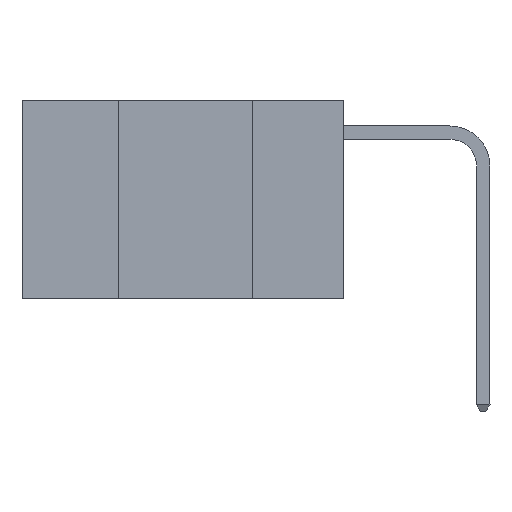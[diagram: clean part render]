
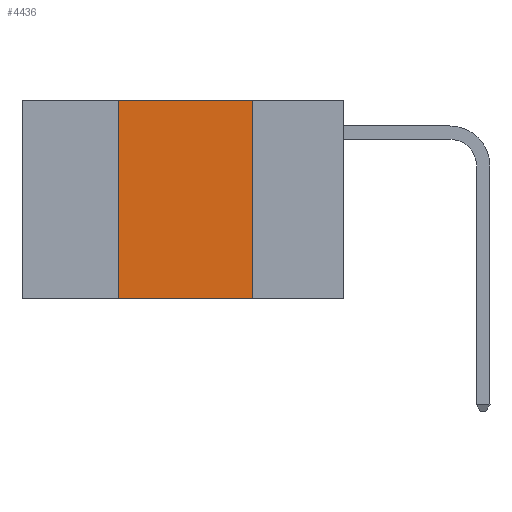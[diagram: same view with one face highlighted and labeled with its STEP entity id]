
A CAD part, left-side view. The second image highlights one B-rep face of the part: STEP entity #4436.
In plain terms, the highlighted planar face has unit normal (-1, 0, 0).
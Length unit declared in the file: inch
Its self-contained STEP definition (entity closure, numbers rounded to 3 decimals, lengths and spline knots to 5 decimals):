
#454 = VECTOR ( 'NONE', #3137, 39.37008 ) ;
#1437 = ORIENTED_EDGE ( 'NONE', *, *, #11161, .F. ) ;
#1546 = DIRECTION ( 'NONE',  ( 1., 0., 0. ) ) ;
#2409 = CARTESIAN_POINT ( 'NONE',  ( 0., 0.6, 0. ) ) ;
#3137 = DIRECTION ( 'NONE',  ( 0., 0., -1. ) ) ;
#3582 = PLANE ( 'NONE',  #13447 ) ;
#3791 = EDGE_CURVE ( 'NONE', #14236, #11285, #14000, .T. ) ;
#4227 = LINE ( 'NONE', #8751, #454 ) ;
#4436 = ADVANCED_FACE ( 'NONE', ( #5826 ), #3582, .F. ) ;
#4669 = DIRECTION ( 'NONE',  ( 0., -1., 0. ) ) ;
#4874 = EDGE_LOOP ( 'NONE', ( #9158, #1437, #14368, #13992 ) ) ;
#5405 = CARTESIAN_POINT ( 'NONE',  ( 0., 0.42, -0.37 ) ) ;
#5416 = EDGE_CURVE ( 'NONE', #14236, #5866, #11280, .T. ) ;
#5826 = FACE_OUTER_BOUND ( 'NONE', #4874, .T. ) ;
#5866 = VERTEX_POINT ( 'NONE', #7673 ) ;
#6348 = VECTOR ( 'NONE', #9938, 39.37008 ) ;
#7673 = CARTESIAN_POINT ( 'NONE',  ( 0., 0.17, -0.37 ) ) ;
#7950 = LINE ( 'NONE', #2409, #9316 ) ;
#8751 = CARTESIAN_POINT ( 'NONE',  ( 0., 0.17, 0. ) ) ;
#9158 = ORIENTED_EDGE ( 'NONE', *, *, #10099, .F. ) ;
#9316 = VECTOR ( 'NONE', #4669, 39.37008 ) ;
#9417 = DIRECTION ( 'NONE',  ( 0., 0., -1. ) ) ;
#9746 = CARTESIAN_POINT ( 'NONE',  ( 0., 0.42, 0. ) ) ;
#9938 = DIRECTION ( 'NONE',  ( 0., -1., 0. ) ) ;
#10099 = EDGE_CURVE ( 'NONE', #14164, #5866, #4227, .T. ) ;
#11066 = CARTESIAN_POINT ( 'NONE',  ( 0., 0.6, -0.37 ) ) ;
#11161 = EDGE_CURVE ( 'NONE', #11285, #14164, #7950, .T. ) ;
#11280 = LINE ( 'NONE', #11066, #6348 ) ;
#11285 = VERTEX_POINT ( 'NONE', #11629 ) ;
#11372 = CARTESIAN_POINT ( 'NONE',  ( 0., 0.17, 0. ) ) ;
#11629 = CARTESIAN_POINT ( 'NONE',  ( 0., 0.42, 0. ) ) ;
#12014 = DIRECTION ( 'NONE',  ( 0., 0., 1. ) ) ;
#13447 = AXIS2_PLACEMENT_3D ( 'NONE', #13594, #1546, #9417 ) ;
#13594 = CARTESIAN_POINT ( 'NONE',  ( 0., 0.6, 0. ) ) ;
#13696 = VECTOR ( 'NONE', #12014, 39.37008 ) ;
#13992 = ORIENTED_EDGE ( 'NONE', *, *, #5416, .T. ) ;
#14000 = LINE ( 'NONE', #9746, #13696 ) ;
#14164 = VERTEX_POINT ( 'NONE', #11372 ) ;
#14236 = VERTEX_POINT ( 'NONE', #5405 ) ;
#14368 = ORIENTED_EDGE ( 'NONE', *, *, #3791, .F. ) ;
